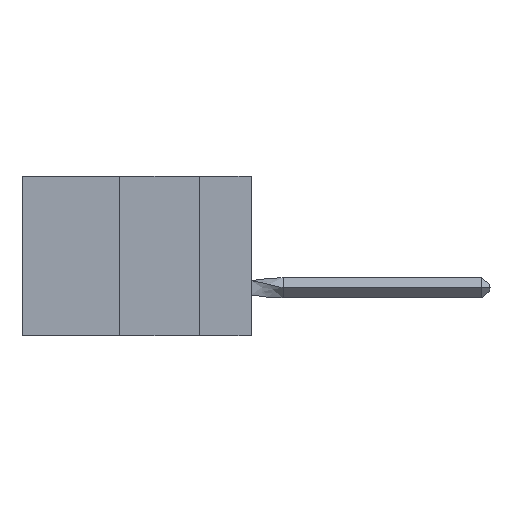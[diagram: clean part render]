
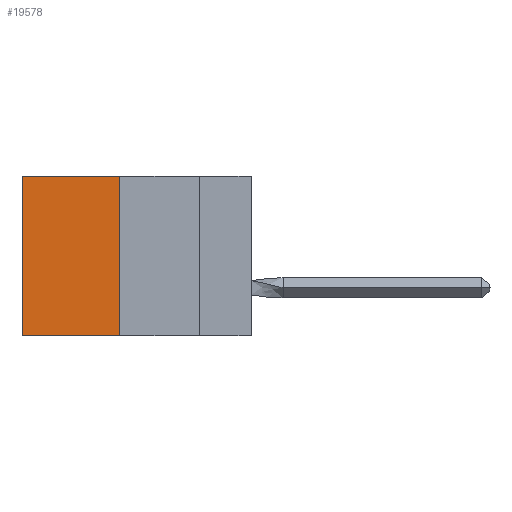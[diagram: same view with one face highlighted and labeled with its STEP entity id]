
A CAD part, left-side view. The second image highlights one B-rep face of the part: STEP entity #19578.
In plain terms, the highlighted planar face has unit normal (-1, 0, 0).
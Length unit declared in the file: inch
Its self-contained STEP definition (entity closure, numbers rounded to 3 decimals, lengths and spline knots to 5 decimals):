
#667 = VERTEX_POINT ( 'NONE', #19983 ) ;
#2128 = DIRECTION ( 'NONE',  ( 0., 0., -1. ) ) ;
#2327 = CARTESIAN_POINT ( 'NONE',  ( 0.305, 0.413, -0.5 ) ) ;
#3100 = VECTOR ( 'NONE', #17511, 39.37008 ) ;
#3226 = VERTEX_POINT ( 'NONE', #2327 ) ;
#4635 = CARTESIAN_POINT ( 'NONE',  ( 0.305, 0.413, 0. ) ) ;
#4876 = LINE ( 'NONE', #10259, #28643 ) ;
#4894 = VERTEX_POINT ( 'NONE', #16750 ) ;
#6888 = LINE ( 'NONE', #24078, #24337 ) ;
#7174 = ORIENTED_EDGE ( 'NONE', *, *, #19982, .F. ) ;
#8104 = ORIENTED_EDGE ( 'NONE', *, *, #25462, .T. ) ;
#10259 = CARTESIAN_POINT ( 'NONE',  ( 0.305, 0.72, -0.5 ) ) ;
#10594 = CARTESIAN_POINT ( 'NONE',  ( 0.305, 0.413, -0.5 ) ) ;
#10844 = CARTESIAN_POINT ( 'NONE',  ( 0.305, 0.413, 0. ) ) ;
#11235 = PLANE ( 'NONE',  #28957 ) ;
#11338 = EDGE_CURVE ( 'NONE', #20674, #3226, #6888, .T. ) ;
#11409 = ORIENTED_EDGE ( 'NONE', *, *, #11338, .F. ) ;
#11530 = CARTESIAN_POINT ( 'NONE',  ( 0.305, 0.413, -0.5 ) ) ;
#14776 = DIRECTION ( 'NONE',  ( 0., 0., -1. ) ) ;
#15933 = DIRECTION ( 'NONE',  ( 1., 0., 0. ) ) ;
#16750 = CARTESIAN_POINT ( 'NONE',  ( 0.305, 0.72, -0.5 ) ) ;
#17072 = LINE ( 'NONE', #10594, #3100 ) ;
#17433 = FACE_OUTER_BOUND ( 'NONE', #27966, .T. ) ;
#17511 = DIRECTION ( 'NONE',  ( 0., 1., 0. ) ) ;
#18165 = LINE ( 'NONE', #4635, #27960 ) ;
#19350 = EDGE_CURVE ( 'NONE', #667, #4894, #4876, .T. ) ;
#19578 = ADVANCED_FACE ( 'NONE', ( #17433 ), #11235, .F. ) ;
#19982 = EDGE_CURVE ( 'NONE', #3226, #4894, #17072, .T. ) ;
#19983 = CARTESIAN_POINT ( 'NONE',  ( 0.305, 0.72, 0. ) ) ;
#20409 = DIRECTION ( 'NONE',  ( 0., 1., 0. ) ) ;
#20572 = DIRECTION ( 'NONE',  ( 0., 0., -1. ) ) ;
#20674 = VERTEX_POINT ( 'NONE', #10844 ) ;
#24078 = CARTESIAN_POINT ( 'NONE',  ( 0.305, 0.413, -0.5 ) ) ;
#24337 = VECTOR ( 'NONE', #2128, 39.37008 ) ;
#25462 = EDGE_CURVE ( 'NONE', #20674, #667, #18165, .T. ) ;
#26550 = ORIENTED_EDGE ( 'NONE', *, *, #19350, .T. ) ;
#27960 = VECTOR ( 'NONE', #20409, 39.37008 ) ;
#27966 = EDGE_LOOP ( 'NONE', ( #26550, #7174, #11409, #8104 ) ) ;
#28643 = VECTOR ( 'NONE', #14776, 39.37008 ) ;
#28957 = AXIS2_PLACEMENT_3D ( 'NONE', #11530, #15933, #20572 ) ;
